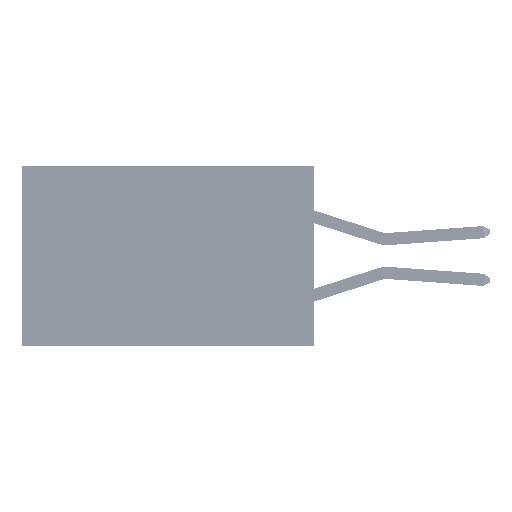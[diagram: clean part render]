
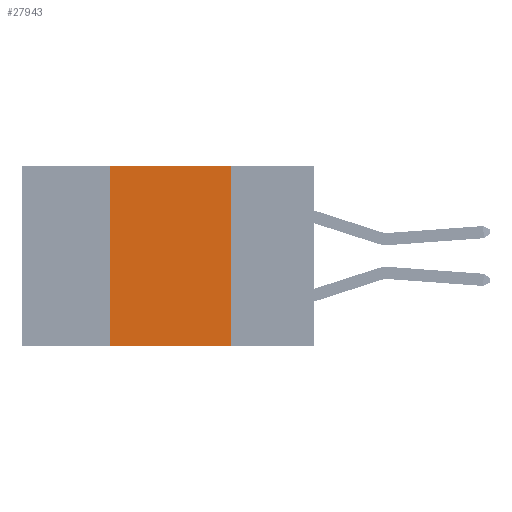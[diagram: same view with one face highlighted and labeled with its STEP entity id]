
A CAD part, left-side view. The second image highlights one B-rep face of the part: STEP entity #27943.
In plain terms, the highlighted planar face has unit normal (-1, 0, 0).
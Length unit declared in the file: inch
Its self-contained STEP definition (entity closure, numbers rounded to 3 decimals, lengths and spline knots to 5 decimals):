
#233 = DIRECTION ( 'NONE',  ( 1., 0., 0. ) ) ;
#1018 = CARTESIAN_POINT ( 'NONE',  ( 0., 0.17, 0. ) ) ;
#1148 = EDGE_LOOP ( 'NONE', ( #19262, #19786, #39110, #35860 ) ) ;
#5671 = VERTEX_POINT ( 'NONE', #14583 ) ;
#6863 = DIRECTION ( 'NONE',  ( 0., 0., 1. ) ) ;
#7151 = CARTESIAN_POINT ( 'NONE',  ( 0., 0.6, -0.37 ) ) ;
#10025 = CARTESIAN_POINT ( 'NONE',  ( 0., 0.42, 0. ) ) ;
#11883 = VECTOR ( 'NONE', #28261, 39.37008 ) ;
#12387 = CARTESIAN_POINT ( 'NONE',  ( 0., 0.17, -0.37 ) ) ;
#12470 = LINE ( 'NONE', #48268, #11883 ) ;
#13777 = DIRECTION ( 'NONE',  ( 0., 0., -1. ) ) ;
#14583 = CARTESIAN_POINT ( 'NONE',  ( 0., 0.42, -0.37 ) ) ;
#18356 = FACE_OUTER_BOUND ( 'NONE', #1148, .T. ) ;
#19089 = VECTOR ( 'NONE', #13777, 39.37008 ) ;
#19262 = ORIENTED_EDGE ( 'NONE', *, *, #39748, .F. ) ;
#19786 = ORIENTED_EDGE ( 'NONE', *, *, #37587, .F. ) ;
#22132 = VERTEX_POINT ( 'NONE', #12387 ) ;
#23885 = CARTESIAN_POINT ( 'NONE',  ( 0., 0.6, 0. ) ) ;
#27943 = ADVANCED_FACE ( 'NONE', ( #18356 ), #39476, .F. ) ;
#28261 = DIRECTION ( 'NONE',  ( 0., -1., 0. ) ) ;
#28460 = EDGE_CURVE ( 'NONE', #5671, #46909, #33626, .T. ) ;
#29333 = VECTOR ( 'NONE', #6863, 39.37008 ) ;
#31772 = EDGE_CURVE ( 'NONE', #5671, #22132, #35020, .T. ) ;
#33626 = LINE ( 'NONE', #49884, #29333 ) ;
#35020 = LINE ( 'NONE', #7151, #50279 ) ;
#35764 = VERTEX_POINT ( 'NONE', #1018 ) ;
#35860 = ORIENTED_EDGE ( 'NONE', *, *, #31772, .T. ) ;
#37587 = EDGE_CURVE ( 'NONE', #46909, #35764, #12470, .T. ) ;
#38081 = LINE ( 'NONE', #45137, #19089 ) ;
#39110 = ORIENTED_EDGE ( 'NONE', *, *, #28460, .F. ) ;
#39476 = PLANE ( 'NONE',  #46467 ) ;
#39748 = EDGE_CURVE ( 'NONE', #35764, #22132, #38081, .T. ) ;
#42433 = DIRECTION ( 'NONE',  ( 0., -1., 0. ) ) ;
#45137 = CARTESIAN_POINT ( 'NONE',  ( 0., 0.17, 0. ) ) ;
#46467 = AXIS2_PLACEMENT_3D ( 'NONE', #23885, #233, #47192 ) ;
#46909 = VERTEX_POINT ( 'NONE', #10025 ) ;
#47192 = DIRECTION ( 'NONE',  ( 0., 0., -1. ) ) ;
#48268 = CARTESIAN_POINT ( 'NONE',  ( 0., 0.6, 0. ) ) ;
#49884 = CARTESIAN_POINT ( 'NONE',  ( 0., 0.42, 0. ) ) ;
#50279 = VECTOR ( 'NONE', #42433, 39.37008 ) ;
